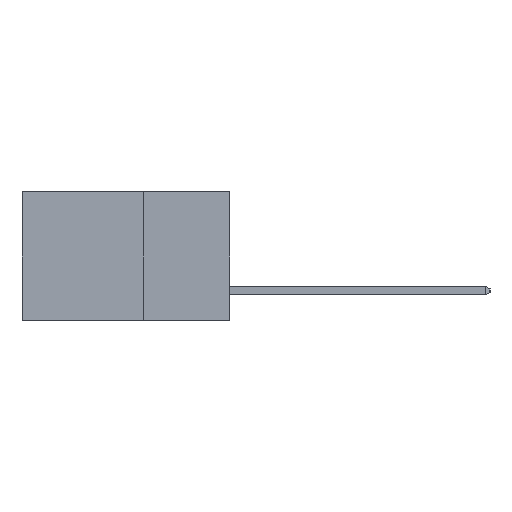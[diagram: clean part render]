
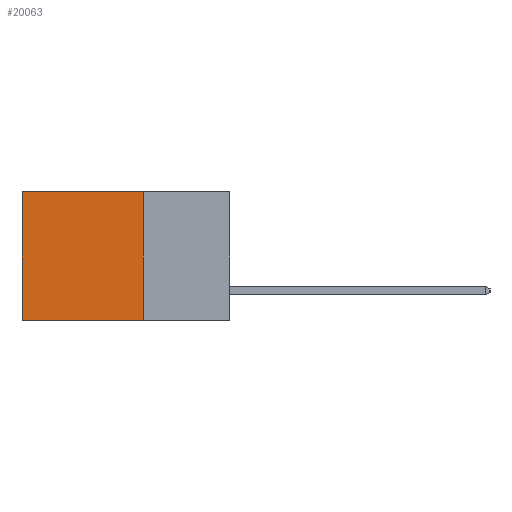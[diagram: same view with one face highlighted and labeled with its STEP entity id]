
A CAD part, left-side view. The second image highlights one B-rep face of the part: STEP entity #20063.
In plain terms, the highlighted planar face has unit normal (-1, 0, 0).
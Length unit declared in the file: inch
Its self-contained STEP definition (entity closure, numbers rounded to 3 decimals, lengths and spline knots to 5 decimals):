
#455 = VECTOR ( 'NONE', #11408, 39.37008 ) ;
#1846 = LINE ( 'NONE', #2918, #21810 ) ;
#1916 = LINE ( 'NONE', #21875, #2493 ) ;
#2493 = VECTOR ( 'NONE', #6301, 39.37008 ) ;
#2918 = CARTESIAN_POINT ( 'NONE',  ( 0.2615, 0.6, -0.37 ) ) ;
#4313 = EDGE_CURVE ( 'NONE', #21950, #23204, #8392, .T. ) ;
#5483 = VERTEX_POINT ( 'NONE', #20275 ) ;
#6301 = DIRECTION ( 'NONE',  ( 0., 0., -1. ) ) ;
#6976 = ORIENTED_EDGE ( 'NONE', *, *, #4313, .F. ) ;
#7161 = ORIENTED_EDGE ( 'NONE', *, *, #13150, .T. ) ;
#7344 = DIRECTION ( 'NONE',  ( 1., 0., 0. ) ) ;
#7656 = CARTESIAN_POINT ( 'NONE',  ( 0.2615, 0.25, -0.37 ) ) ;
#8392 = LINE ( 'NONE', #22761, #23275 ) ;
#9122 = CARTESIAN_POINT ( 'NONE',  ( 0.2615, 0.25, -0.37 ) ) ;
#9453 = CARTESIAN_POINT ( 'NONE',  ( 0.2615, 0.25, 0. ) ) ;
#9683 = VERTEX_POINT ( 'NONE', #22709 ) ;
#9880 = CARTESIAN_POINT ( 'NONE',  ( 0.2615, 0.6, -0.37 ) ) ;
#10141 = EDGE_CURVE ( 'NONE', #9683, #5483, #15871, .T. ) ;
#11408 = DIRECTION ( 'NONE',  ( 0., 1., 0. ) ) ;
#13150 = EDGE_CURVE ( 'NONE', #5483, #23204, #1846, .T. ) ;
#15716 = ORIENTED_EDGE ( 'NONE', *, *, #10141, .T. ) ;
#15871 = LINE ( 'NONE', #9453, #455 ) ;
#16106 = EDGE_CURVE ( 'NONE', #9683, #21950, #1916, .T. ) ;
#17056 = DIRECTION ( 'NONE',  ( 0., 1., 0. ) ) ;
#17831 = FACE_OUTER_BOUND ( 'NONE', #20160, .T. ) ;
#18704 = AXIS2_PLACEMENT_3D ( 'NONE', #9122, #7344, #20961 ) ;
#19022 = ORIENTED_EDGE ( 'NONE', *, *, #16106, .F. ) ;
#19026 = PLANE ( 'NONE',  #18704 ) ;
#20063 = ADVANCED_FACE ( 'NONE', ( #17831 ), #19026, .F. ) ;
#20160 = EDGE_LOOP ( 'NONE', ( #7161, #6976, #19022, #15716 ) ) ;
#20275 = CARTESIAN_POINT ( 'NONE',  ( 0.2615, 0.6, 0. ) ) ;
#20961 = DIRECTION ( 'NONE',  ( 0., 0., -1. ) ) ;
#21810 = VECTOR ( 'NONE', #24202, 39.37008 ) ;
#21875 = CARTESIAN_POINT ( 'NONE',  ( 0.2615, 0.25, -0.37 ) ) ;
#21950 = VERTEX_POINT ( 'NONE', #7656 ) ;
#22709 = CARTESIAN_POINT ( 'NONE',  ( 0.2615, 0.25, 0. ) ) ;
#22761 = CARTESIAN_POINT ( 'NONE',  ( 0.2615, 0.25, -0.37 ) ) ;
#23204 = VERTEX_POINT ( 'NONE', #9880 ) ;
#23275 = VECTOR ( 'NONE', #17056, 39.37008 ) ;
#24202 = DIRECTION ( 'NONE',  ( 0., 0., -1. ) ) ;
